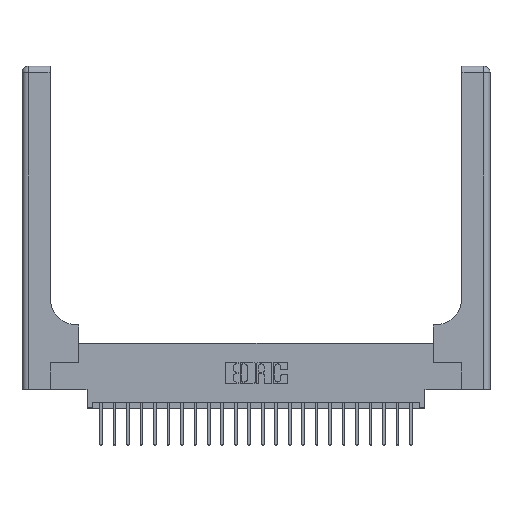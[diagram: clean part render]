
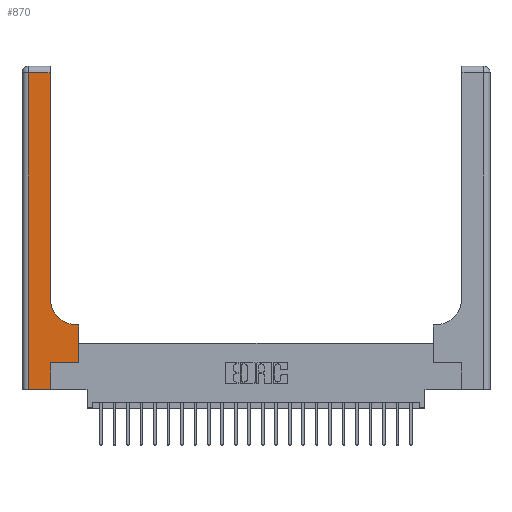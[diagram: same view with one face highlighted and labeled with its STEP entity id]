
A CAD part, top view. The second image highlights one B-rep face of the part: STEP entity #870.
In plain terms, the highlighted planar face has unit normal (0, 0, 1).
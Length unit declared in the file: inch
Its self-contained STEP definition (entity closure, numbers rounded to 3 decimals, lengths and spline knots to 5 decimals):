
#56 = DIRECTION ( 'NONE',  ( 1., 0., 0. ) ) ;
#433 = VECTOR ( 'NONE', #4170, 39.37008 ) ;
#665 = EDGE_CURVE ( 'NONE', #13978, #18424, #22698, .T. ) ;
#870 = ADVANCED_FACE ( 'NONE', ( #15584 ), #2756, .F. ) ;
#1146 = EDGE_CURVE ( 'NONE', #3037, #12968, #20522, .T. ) ;
#1630 = VERTEX_POINT ( 'NONE', #4836 ) ;
#2756 = PLANE ( 'NONE',  #16796 ) ;
#3037 = VERTEX_POINT ( 'NONE', #9106 ) ;
#3276 = EDGE_CURVE ( 'NONE', #15678, #3037, #7427, .T. ) ;
#3434 = EDGE_LOOP ( 'NONE', ( #14171, #9220, #8329, #16609, #19851, #18862, #10808, #18675, #20552 ) ) ;
#3445 = CARTESIAN_POINT ( 'NONE',  ( 0., 0., 0.37 ) ) ;
#3517 = VERTEX_POINT ( 'NONE', #22873 ) ;
#3685 = VECTOR ( 'NONE', #17048, 39.37008 ) ;
#3826 = LINE ( 'NONE', #12900, #16824 ) ;
#3944 = CARTESIAN_POINT ( 'NONE',  ( 0.265, 0., 0.37 ) ) ;
#4170 = DIRECTION ( 'NONE',  ( -1., 0., 0. ) ) ;
#4414 = AXIS2_PLACEMENT_3D ( 'NONE', #7073, #20246, #14454 ) ;
#4673 = EDGE_CURVE ( 'NONE', #11243, #3517, #3826, .T. ) ;
#4814 = CARTESIAN_POINT ( 'NONE',  ( 0.06, 0., 0.37 ) ) ;
#4836 = CARTESIAN_POINT ( 'NONE',  ( 0.51, 0.6, 0.37 ) ) ;
#5468 = LINE ( 'NONE', #23592, #7161 ) ;
#5601 = CARTESIAN_POINT ( 'NONE',  ( 0., 2.94, 0.37 ) ) ;
#7073 = CARTESIAN_POINT ( 'NONE',  ( 0.51, 0.85, 0.37 ) ) ;
#7161 = VECTOR ( 'NONE', #18285, 39.37008 ) ;
#7371 = DIRECTION ( 'NONE',  ( 0., -1., 0. ) ) ;
#7427 = LINE ( 'NONE', #3445, #9780 ) ;
#7568 = CARTESIAN_POINT ( 'NONE',  ( 0.265, 0.25, 0.37 ) ) ;
#7583 = DIRECTION ( 'NONE',  ( 0., 1., 0. ) ) ;
#8091 = CARTESIAN_POINT ( 'NONE',  ( 0.26, 3., 0.37 ) ) ;
#8329 = ORIENTED_EDGE ( 'NONE', *, *, #18223, .T. ) ;
#8556 = VECTOR ( 'NONE', #7371, 39.37008 ) ;
#8817 = CARTESIAN_POINT ( 'NONE',  ( 0.06, 3., 0.37 ) ) ;
#8943 = LINE ( 'NONE', #8817, #8556 ) ;
#9106 = CARTESIAN_POINT ( 'NONE',  ( 0.265, 0., 0.37 ) ) ;
#9131 = CARTESIAN_POINT ( 'NONE',  ( 0.528, 0.25, 0.37 ) ) ;
#9220 = ORIENTED_EDGE ( 'NONE', *, *, #13360, .T. ) ;
#9780 = VECTOR ( 'NONE', #56, 39.37008 ) ;
#10390 = DIRECTION ( 'NONE',  ( 0., 0., -1. ) ) ;
#10808 = ORIENTED_EDGE ( 'NONE', *, *, #4673, .T. ) ;
#10926 = CARTESIAN_POINT ( 'NONE',  ( 0.06, 2.94, 0.37 ) ) ;
#11243 = VERTEX_POINT ( 'NONE', #9131 ) ;
#12900 = CARTESIAN_POINT ( 'NONE',  ( 0.528, 0.25, 0.37 ) ) ;
#12968 = VERTEX_POINT ( 'NONE', #7568 ) ;
#13005 = LINE ( 'NONE', #17119, #433 ) ;
#13360 = EDGE_CURVE ( 'NONE', #18424, #20533, #16494, .T. ) ;
#13978 = VERTEX_POINT ( 'NONE', #15602 ) ;
#14171 = ORIENTED_EDGE ( 'NONE', *, *, #665, .T. ) ;
#14454 = DIRECTION ( 'NONE',  ( 1., 0., 0. ) ) ;
#14728 = DIRECTION ( 'NONE',  ( 0., 1., 0. ) ) ;
#15584 = FACE_OUTER_BOUND ( 'NONE', #3434, .T. ) ;
#15602 = CARTESIAN_POINT ( 'NONE',  ( 0.26, 0.85, 0.37 ) ) ;
#15678 = VERTEX_POINT ( 'NONE', #4814 ) ;
#16494 = LINE ( 'NONE', #5601, #22348 ) ;
#16609 = ORIENTED_EDGE ( 'NONE', *, *, #3276, .T. ) ;
#16796 = AXIS2_PLACEMENT_3D ( 'NONE', #17519, #10390, #21015 ) ;
#16824 = VECTOR ( 'NONE', #14728, 39.37008 ) ;
#17048 = DIRECTION ( 'NONE',  ( 0., 1., 0. ) ) ;
#17119 = CARTESIAN_POINT ( 'NONE',  ( 0.26, 0.6, 0.37 ) ) ;
#17519 = CARTESIAN_POINT ( 'NONE',  ( 0., 3., 0.37 ) ) ;
#17569 = EDGE_CURVE ( 'NONE', #3517, #1630, #13005, .T. ) ;
#18223 = EDGE_CURVE ( 'NONE', #20533, #15678, #8943, .T. ) ;
#18285 = DIRECTION ( 'NONE',  ( 1., 0., 0. ) ) ;
#18424 = VERTEX_POINT ( 'NONE', #18600 ) ;
#18600 = CARTESIAN_POINT ( 'NONE',  ( 0.26, 2.94, 0.37 ) ) ;
#18675 = ORIENTED_EDGE ( 'NONE', *, *, #17569, .T. ) ;
#18720 = CIRCLE ( 'NONE', #4414, 0.25 ) ;
#18862 = ORIENTED_EDGE ( 'NONE', *, *, #22276, .T. ) ;
#18944 = VECTOR ( 'NONE', #7583, 39.37008 ) ;
#19851 = ORIENTED_EDGE ( 'NONE', *, *, #1146, .T. ) ;
#20246 = DIRECTION ( 'NONE',  ( 0., 0., -1. ) ) ;
#20353 = DIRECTION ( 'NONE',  ( -1., 0., 0. ) ) ;
#20522 = LINE ( 'NONE', #3944, #18944 ) ;
#20533 = VERTEX_POINT ( 'NONE', #10926 ) ;
#20552 = ORIENTED_EDGE ( 'NONE', *, *, #21868, .T. ) ;
#21015 = DIRECTION ( 'NONE',  ( -1., 0., 0. ) ) ;
#21868 = EDGE_CURVE ( 'NONE', #1630, #13978, #18720, .T. ) ;
#22276 = EDGE_CURVE ( 'NONE', #12968, #11243, #5468, .T. ) ;
#22348 = VECTOR ( 'NONE', #20353, 39.37008 ) ;
#22698 = LINE ( 'NONE', #8091, #3685 ) ;
#22873 = CARTESIAN_POINT ( 'NONE',  ( 0.528, 0.6, 0.37 ) ) ;
#23592 = CARTESIAN_POINT ( 'NONE',  ( 0.265, 0.25, 0.37 ) ) ;
